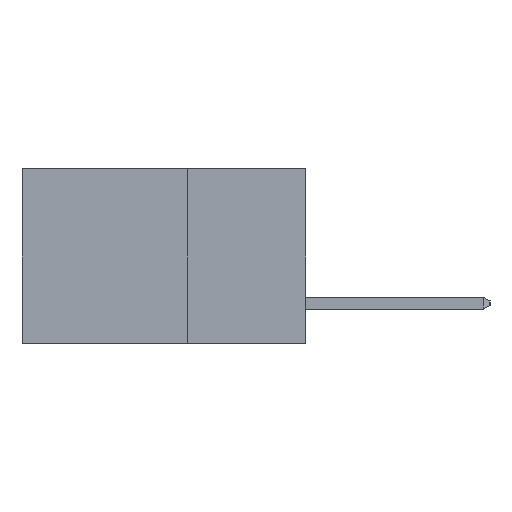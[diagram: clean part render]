
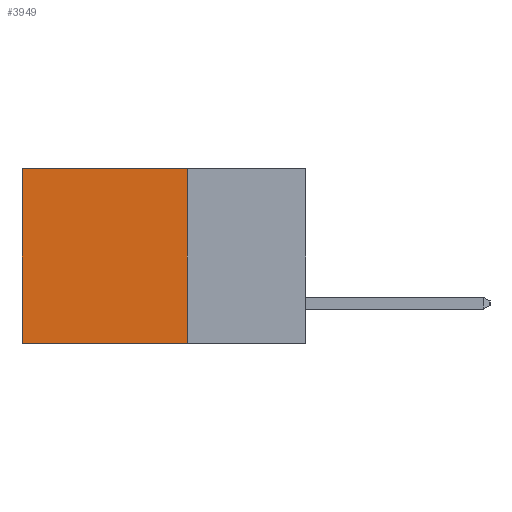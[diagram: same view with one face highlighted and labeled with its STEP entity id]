
A CAD part, left-side view. The second image highlights one B-rep face of the part: STEP entity #3949.
In plain terms, the highlighted planar face has unit normal (-1, 0, 0).
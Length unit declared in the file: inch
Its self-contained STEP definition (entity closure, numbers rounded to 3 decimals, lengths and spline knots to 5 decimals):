
#357 = CARTESIAN_POINT ( 'NONE',  ( 0.2615, 0.6, -0.37 ) ) ;
#388 = DIRECTION ( 'NONE',  ( 0., 0., -1. ) ) ;
#436 = LINE ( 'NONE', #7588, #6226 ) ;
#489 = ORIENTED_EDGE ( 'NONE', *, *, #9596, .F. ) ;
#728 = FACE_OUTER_BOUND ( 'NONE', #3880, .T. ) ;
#855 = VECTOR ( 'NONE', #5419, 39.37008 ) ;
#2285 = DIRECTION ( 'NONE',  ( 0., 0., -1. ) ) ;
#2423 = EDGE_CURVE ( 'NONE', #4088, #3209, #436, .T. ) ;
#2901 = CARTESIAN_POINT ( 'NONE',  ( 0.2615, 0.25, 0. ) ) ;
#3040 = VECTOR ( 'NONE', #2285, 39.37008 ) ;
#3209 = VERTEX_POINT ( 'NONE', #8643 ) ;
#3584 = LINE ( 'NONE', #5519, #855 ) ;
#3662 = EDGE_CURVE ( 'NONE', #8808, #4547, #3584, .T. ) ;
#3705 = DIRECTION ( 'NONE',  ( 0., 0., -1. ) ) ;
#3722 = PLANE ( 'NONE',  #8154 ) ;
#3767 = CARTESIAN_POINT ( 'NONE',  ( 0.2615, 0.25, -0.37 ) ) ;
#3837 = DIRECTION ( 'NONE',  ( 1., 0., 0. ) ) ;
#3880 = EDGE_LOOP ( 'NONE', ( #9401, #9619, #489, #4207 ) ) ;
#3949 = ADVANCED_FACE ( 'NONE', ( #728 ), #3722, .F. ) ;
#4088 = VERTEX_POINT ( 'NONE', #2901 ) ;
#4207 = ORIENTED_EDGE ( 'NONE', *, *, #2423, .T. ) ;
#4547 = VERTEX_POINT ( 'NONE', #8529 ) ;
#4591 = LINE ( 'NONE', #6139, #3040 ) ;
#4711 = VECTOR ( 'NONE', #388, 39.37008 ) ;
#5419 = DIRECTION ( 'NONE',  ( 0., 1., 0. ) ) ;
#5519 = CARTESIAN_POINT ( 'NONE',  ( 0.2615, 0.25, -0.37 ) ) ;
#6139 = CARTESIAN_POINT ( 'NONE',  ( 0.2615, 0.25, -0.37 ) ) ;
#6226 = VECTOR ( 'NONE', #6643, 39.37008 ) ;
#6236 = CARTESIAN_POINT ( 'NONE',  ( 0.2615, 0.25, -0.37 ) ) ;
#6282 = EDGE_CURVE ( 'NONE', #3209, #4547, #6669, .T. ) ;
#6643 = DIRECTION ( 'NONE',  ( 0., 1., 0. ) ) ;
#6669 = LINE ( 'NONE', #357, #4711 ) ;
#7588 = CARTESIAN_POINT ( 'NONE',  ( 0.2615, 0.25, 0. ) ) ;
#8154 = AXIS2_PLACEMENT_3D ( 'NONE', #3767, #3837, #3705 ) ;
#8529 = CARTESIAN_POINT ( 'NONE',  ( 0.2615, 0.6, -0.37 ) ) ;
#8643 = CARTESIAN_POINT ( 'NONE',  ( 0.2615, 0.6, 0. ) ) ;
#8808 = VERTEX_POINT ( 'NONE', #6236 ) ;
#9401 = ORIENTED_EDGE ( 'NONE', *, *, #6282, .T. ) ;
#9596 = EDGE_CURVE ( 'NONE', #4088, #8808, #4591, .T. ) ;
#9619 = ORIENTED_EDGE ( 'NONE', *, *, #3662, .F. ) ;
